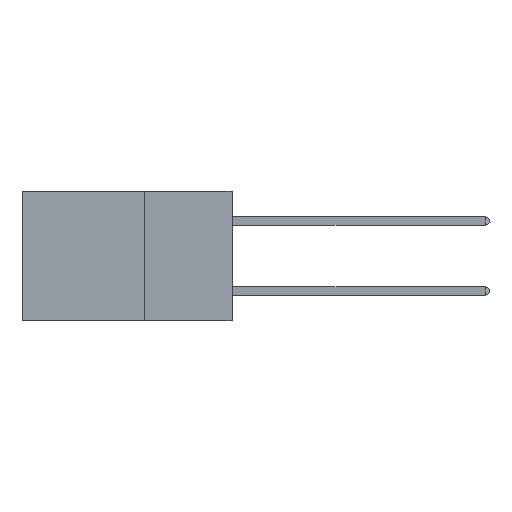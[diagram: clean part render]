
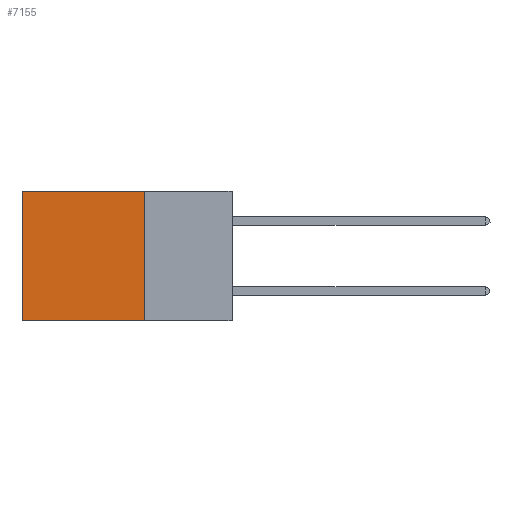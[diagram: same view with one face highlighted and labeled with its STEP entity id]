
A CAD part, left-side view. The second image highlights one B-rep face of the part: STEP entity #7155.
In plain terms, the highlighted planar face has unit normal (-1, 0, 0).
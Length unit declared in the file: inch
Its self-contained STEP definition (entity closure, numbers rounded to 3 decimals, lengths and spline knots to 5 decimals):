
#282 = VERTEX_POINT ( 'NONE', #8555 ) ;
#290 = DIRECTION ( 'NONE',  ( 0., 1., 0. ) ) ;
#478 = CARTESIAN_POINT ( 'NONE',  ( 0.2875, 0.6, 0. ) ) ;
#669 = EDGE_CURVE ( 'NONE', #282, #7443, #15345, .T. ) ;
#711 = VECTOR ( 'NONE', #14684, 39.37008 ) ;
#1095 = EDGE_CURVE ( 'NONE', #7443, #16577, #3040, .T. ) ;
#1117 = CARTESIAN_POINT ( 'NONE',  ( 0.2875, 0.6, 0. ) ) ;
#2788 = LINE ( 'NONE', #10986, #17951 ) ;
#3040 = LINE ( 'NONE', #1117, #11330 ) ;
#3088 = ORIENTED_EDGE ( 'NONE', *, *, #1095, .T. ) ;
#3907 = AXIS2_PLACEMENT_3D ( 'NONE', #15386, #14064, #5122 ) ;
#4645 = LINE ( 'NONE', #13116, #711 ) ;
#4960 = ORIENTED_EDGE ( 'NONE', *, *, #9874, .F. ) ;
#5122 = DIRECTION ( 'NONE',  ( 0., 0., -1. ) ) ;
#6561 = FACE_OUTER_BOUND ( 'NONE', #7200, .T. ) ;
#7155 = ADVANCED_FACE ( 'NONE', ( #6561 ), #8295, .F. ) ;
#7200 = EDGE_LOOP ( 'NONE', ( #3088, #18212, #4960, #7481 ) ) ;
#7443 = VERTEX_POINT ( 'NONE', #478 ) ;
#7481 = ORIENTED_EDGE ( 'NONE', *, *, #669, .T. ) ;
#8127 = VERTEX_POINT ( 'NONE', #9419 ) ;
#8295 = PLANE ( 'NONE',  #3907 ) ;
#8555 = CARTESIAN_POINT ( 'NONE',  ( 0.2875, 0.25, 0. ) ) ;
#9084 = EDGE_CURVE ( 'NONE', #8127, #16577, #4645, .T. ) ;
#9419 = CARTESIAN_POINT ( 'NONE',  ( 0.2875, 0.25, -0.37 ) ) ;
#9874 = EDGE_CURVE ( 'NONE', #282, #8127, #2788, .T. ) ;
#10986 = CARTESIAN_POINT ( 'NONE',  ( 0.2875, 0.25, 0. ) ) ;
#11254 = DIRECTION ( 'NONE',  ( 0., 0., -1. ) ) ;
#11330 = VECTOR ( 'NONE', #15759, 39.37008 ) ;
#12612 = CARTESIAN_POINT ( 'NONE',  ( 0.2875, 0.6, -0.37 ) ) ;
#13116 = CARTESIAN_POINT ( 'NONE',  ( 0.2875, 0.25, -0.37 ) ) ;
#13481 = CARTESIAN_POINT ( 'NONE',  ( 0.2875, 0.25, 0. ) ) ;
#14064 = DIRECTION ( 'NONE',  ( 1., 0., 0. ) ) ;
#14684 = DIRECTION ( 'NONE',  ( 0., 1., 0. ) ) ;
#15345 = LINE ( 'NONE', #13481, #18567 ) ;
#15386 = CARTESIAN_POINT ( 'NONE',  ( 0.2875, 0.25, 0. ) ) ;
#15759 = DIRECTION ( 'NONE',  ( 0., 0., -1. ) ) ;
#16577 = VERTEX_POINT ( 'NONE', #12612 ) ;
#17951 = VECTOR ( 'NONE', #11254, 39.37008 ) ;
#18212 = ORIENTED_EDGE ( 'NONE', *, *, #9084, .F. ) ;
#18567 = VECTOR ( 'NONE', #290, 39.37008 ) ;
